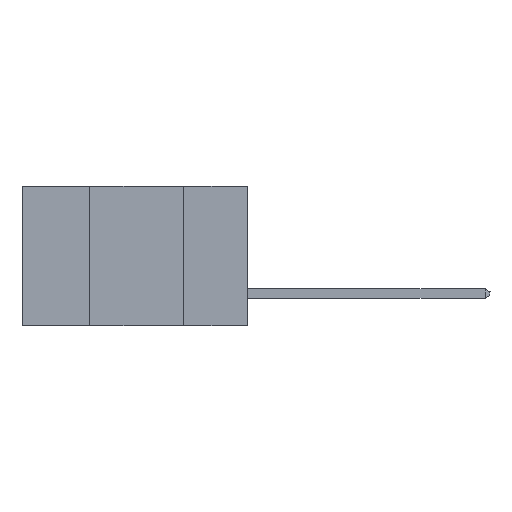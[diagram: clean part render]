
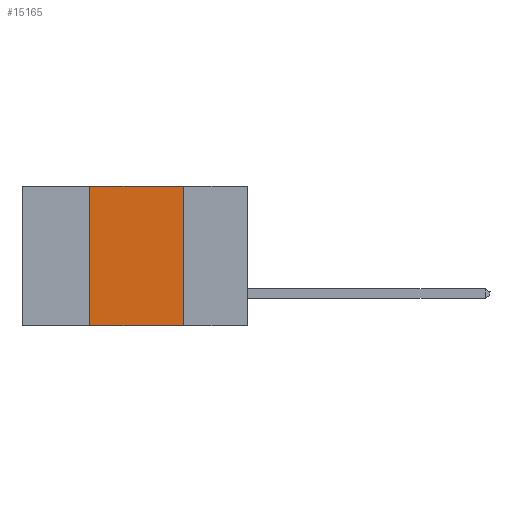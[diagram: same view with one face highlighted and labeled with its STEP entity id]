
A CAD part, left-side view. The second image highlights one B-rep face of the part: STEP entity #15165.
In plain terms, the highlighted planar face has unit normal (-1, 0, 0).
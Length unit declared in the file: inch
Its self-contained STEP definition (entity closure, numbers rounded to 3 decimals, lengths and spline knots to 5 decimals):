
#535 = DIRECTION ( 'NONE',  ( 1., 0., 0. ) ) ;
#1030 = AXIS2_PLACEMENT_3D ( 'NONE', #8500, #535, #9825 ) ;
#1114 = CARTESIAN_POINT ( 'NONE',  ( 0., 0.42, 0. ) ) ;
#1452 = EDGE_LOOP ( 'NONE', ( #6789, #10520, #15199, #5978 ) ) ;
#2621 = CARTESIAN_POINT ( 'NONE',  ( 0., 0.17, -0.37 ) ) ;
#2710 = CARTESIAN_POINT ( 'NONE',  ( 0., 0.17, 0. ) ) ;
#3456 = EDGE_CURVE ( 'NONE', #10666, #5762, #7704, .T. ) ;
#4526 = CARTESIAN_POINT ( 'NONE',  ( 0., 0.6, -0.37 ) ) ;
#4882 = LINE ( 'NONE', #4526, #14656 ) ;
#5166 = DIRECTION ( 'NONE',  ( 0., 0., -1. ) ) ;
#5503 = VECTOR ( 'NONE', #12945, 39.37008 ) ;
#5762 = VERTEX_POINT ( 'NONE', #2621 ) ;
#5978 = ORIENTED_EDGE ( 'NONE', *, *, #13368, .T. ) ;
#6199 = VERTEX_POINT ( 'NONE', #13846 ) ;
#6789 = ORIENTED_EDGE ( 'NONE', *, *, #3456, .F. ) ;
#7143 = PLANE ( 'NONE',  #1030 ) ;
#7199 = LINE ( 'NONE', #1114, #14711 ) ;
#7704 = LINE ( 'NONE', #2710, #17072 ) ;
#7745 = FACE_OUTER_BOUND ( 'NONE', #1452, .T. ) ;
#8500 = CARTESIAN_POINT ( 'NONE',  ( 0., 0.6, 0. ) ) ;
#8880 = CARTESIAN_POINT ( 'NONE',  ( 0., 0.6, 0. ) ) ;
#9401 = EDGE_CURVE ( 'NONE', #12526, #6199, #7199, .T. ) ;
#9825 = DIRECTION ( 'NONE',  ( 0., 0., -1. ) ) ;
#10520 = ORIENTED_EDGE ( 'NONE', *, *, #13495, .F. ) ;
#10666 = VERTEX_POINT ( 'NONE', #16435 ) ;
#11332 = DIRECTION ( 'NONE',  ( 0., -1., 0. ) ) ;
#12526 = VERTEX_POINT ( 'NONE', #15280 ) ;
#12945 = DIRECTION ( 'NONE',  ( 0., -1., 0. ) ) ;
#13368 = EDGE_CURVE ( 'NONE', #12526, #5762, #4882, .T. ) ;
#13495 = EDGE_CURVE ( 'NONE', #6199, #10666, #14232, .T. ) ;
#13846 = CARTESIAN_POINT ( 'NONE',  ( 0., 0.42, 0. ) ) ;
#14232 = LINE ( 'NONE', #8880, #5503 ) ;
#14656 = VECTOR ( 'NONE', #11332, 39.37008 ) ;
#14711 = VECTOR ( 'NONE', #15905, 39.37008 ) ;
#15165 = ADVANCED_FACE ( 'NONE', ( #7745 ), #7143, .F. ) ;
#15199 = ORIENTED_EDGE ( 'NONE', *, *, #9401, .F. ) ;
#15280 = CARTESIAN_POINT ( 'NONE',  ( 0., 0.42, -0.37 ) ) ;
#15905 = DIRECTION ( 'NONE',  ( 0., 0., 1. ) ) ;
#16435 = CARTESIAN_POINT ( 'NONE',  ( 0., 0.17, 0. ) ) ;
#17072 = VECTOR ( 'NONE', #5166, 39.37008 ) ;
